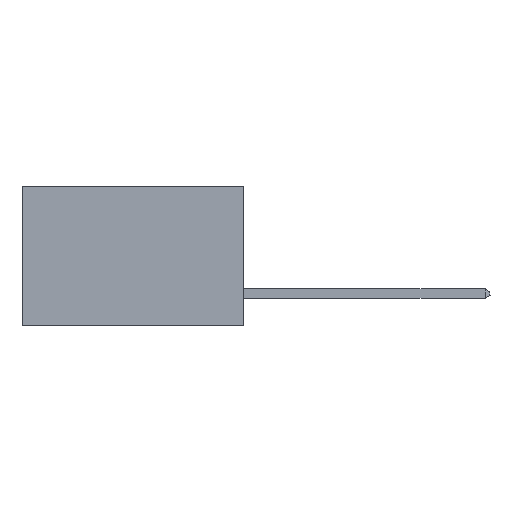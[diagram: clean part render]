
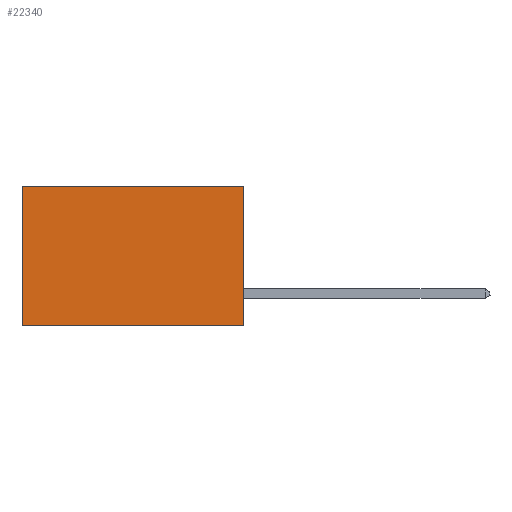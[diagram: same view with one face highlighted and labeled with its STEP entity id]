
A CAD part, left-side view. The second image highlights one B-rep face of the part: STEP entity #22340.
In plain terms, the highlighted planar face has unit normal (-1, 0, 0).
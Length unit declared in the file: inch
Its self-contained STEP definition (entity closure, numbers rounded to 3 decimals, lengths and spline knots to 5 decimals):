
#83 = DIRECTION ( 'NONE',  ( 0., 0., -1. ) ) ;
#90 = VERTEX_POINT ( 'NONE', #18040 ) ;
#101 = FACE_OUTER_BOUND ( 'NONE', #13897, .T. ) ;
#656 = DIRECTION ( 'NONE',  ( 0., 1., 0. ) ) ;
#1039 = CARTESIAN_POINT ( 'NONE',  ( 0.277, 0.59, 0. ) ) ;
#1172 = VECTOR ( 'NONE', #656, 39.37008 ) ;
#1246 = LINE ( 'NONE', #13306, #14181 ) ;
#1944 = LINE ( 'NONE', #5391, #11839 ) ;
#2359 = ORIENTED_EDGE ( 'NONE', *, *, #14843, .T. ) ;
#2819 = AXIS2_PLACEMENT_3D ( 'NONE', #8884, #10632, #83 ) ;
#4774 = VERTEX_POINT ( 'NONE', #15214 ) ;
#5391 = CARTESIAN_POINT ( 'NONE',  ( 0.277, 0.59, -0.37 ) ) ;
#7160 = DIRECTION ( 'NONE',  ( 0., 0., -1. ) ) ;
#8625 = EDGE_CURVE ( 'NONE', #14891, #90, #12474, .T. ) ;
#8884 = CARTESIAN_POINT ( 'NONE',  ( 0.277, 0., -0.37 ) ) ;
#10557 = LINE ( 'NONE', #21419, #1172 ) ;
#10632 = DIRECTION ( 'NONE',  ( 1., 0., 0. ) ) ;
#11387 = VERTEX_POINT ( 'NONE', #1039 ) ;
#11408 = ORIENTED_EDGE ( 'NONE', *, *, #8625, .F. ) ;
#11839 = VECTOR ( 'NONE', #7160, 39.37008 ) ;
#12355 = EDGE_CURVE ( 'NONE', #11387, #4774, #1944, .T. ) ;
#12474 = LINE ( 'NONE', #16037, #20486 ) ;
#13306 = CARTESIAN_POINT ( 'NONE',  ( 0.277, 0., 0. ) ) ;
#13714 = ORIENTED_EDGE ( 'NONE', *, *, #12355, .T. ) ;
#13897 = EDGE_LOOP ( 'NONE', ( #13714, #16847, #11408, #2359 ) ) ;
#14181 = VECTOR ( 'NONE', #15056, 39.37008 ) ;
#14843 = EDGE_CURVE ( 'NONE', #14891, #11387, #1246, .T. ) ;
#14891 = VERTEX_POINT ( 'NONE', #16891 ) ;
#15056 = DIRECTION ( 'NONE',  ( 0., 1., 0. ) ) ;
#15214 = CARTESIAN_POINT ( 'NONE',  ( 0.277, 0.59, -0.37 ) ) ;
#15867 = DIRECTION ( 'NONE',  ( 0., 0., -1. ) ) ;
#16037 = CARTESIAN_POINT ( 'NONE',  ( 0.277, 0., -0.37 ) ) ;
#16739 = EDGE_CURVE ( 'NONE', #90, #4774, #10557, .T. ) ;
#16847 = ORIENTED_EDGE ( 'NONE', *, *, #16739, .F. ) ;
#16891 = CARTESIAN_POINT ( 'NONE',  ( 0.277, 0., 0. ) ) ;
#18040 = CARTESIAN_POINT ( 'NONE',  ( 0.277, 0., -0.37 ) ) ;
#19177 = PLANE ( 'NONE',  #2819 ) ;
#20486 = VECTOR ( 'NONE', #15867, 39.37008 ) ;
#21419 = CARTESIAN_POINT ( 'NONE',  ( 0.277, 0., -0.37 ) ) ;
#22340 = ADVANCED_FACE ( 'NONE', ( #101 ), #19177, .F. ) ;
